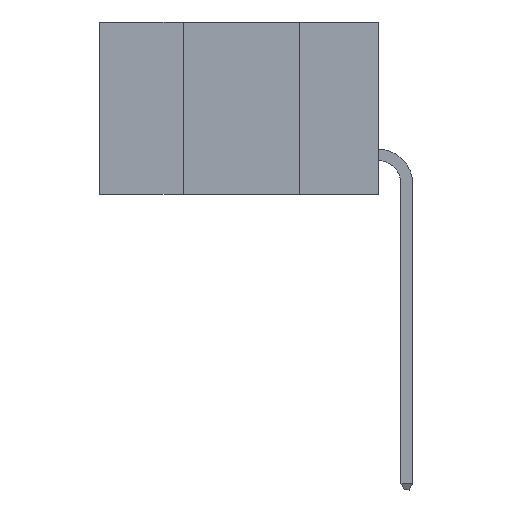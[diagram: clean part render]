
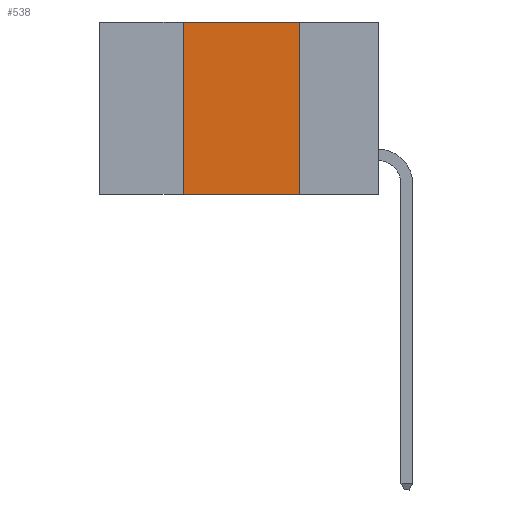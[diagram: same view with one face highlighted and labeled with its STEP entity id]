
A CAD part, left-side view. The second image highlights one B-rep face of the part: STEP entity #538.
In plain terms, the highlighted planar face has unit normal (-1, 0, 0).
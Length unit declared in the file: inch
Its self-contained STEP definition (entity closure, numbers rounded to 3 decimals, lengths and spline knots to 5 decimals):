
#421 = EDGE_LOOP ( 'NONE', ( #5904, #5609, #13743, #13166 ) ) ;
#538 = ADVANCED_FACE ( 'NONE', ( #7752 ), #2664, .F. ) ;
#1612 = CARTESIAN_POINT ( 'NONE',  ( 0., 0.17, 0. ) ) ;
#2026 = VECTOR ( 'NONE', #13033, 39.37008 ) ;
#2372 = DIRECTION ( 'NONE',  ( 0., -1., 0. ) ) ;
#2664 = PLANE ( 'NONE',  #4164 ) ;
#3254 = VERTEX_POINT ( 'NONE', #11123 ) ;
#3627 = EDGE_CURVE ( 'NONE', #9568, #3254, #14555, .T. ) ;
#3674 = DIRECTION ( 'NONE',  ( 0., 0., -1. ) ) ;
#4120 = VECTOR ( 'NONE', #5098, 39.37008 ) ;
#4164 = AXIS2_PLACEMENT_3D ( 'NONE', #4630, #5545, #3674 ) ;
#4630 = CARTESIAN_POINT ( 'NONE',  ( 0., 0.6, 0. ) ) ;
#5098 = DIRECTION ( 'NONE',  ( 0., 0., -1. ) ) ;
#5545 = DIRECTION ( 'NONE',  ( 1., 0., 0. ) ) ;
#5562 = DIRECTION ( 'NONE',  ( 0., -1., 0. ) ) ;
#5609 = ORIENTED_EDGE ( 'NONE', *, *, #7750, .F. ) ;
#5904 = ORIENTED_EDGE ( 'NONE', *, *, #6982, .F. ) ;
#6234 = EDGE_CURVE ( 'NONE', #9568, #12731, #7183, .T. ) ;
#6982 = EDGE_CURVE ( 'NONE', #8669, #12731, #11295, .T. ) ;
#7183 = LINE ( 'NONE', #10643, #13020 ) ;
#7711 = CARTESIAN_POINT ( 'NONE',  ( 0., 0.42, -0.37 ) ) ;
#7750 = EDGE_CURVE ( 'NONE', #3254, #8669, #12399, .T. ) ;
#7752 = FACE_OUTER_BOUND ( 'NONE', #421, .T. ) ;
#7770 = CARTESIAN_POINT ( 'NONE',  ( 0., 0.42, 0. ) ) ;
#8669 = VERTEX_POINT ( 'NONE', #11096 ) ;
#9568 = VERTEX_POINT ( 'NONE', #7711 ) ;
#10643 = CARTESIAN_POINT ( 'NONE',  ( 0., 0.6, -0.37 ) ) ;
#10665 = CARTESIAN_POINT ( 'NONE',  ( 0., 0.17, -0.37 ) ) ;
#10879 = CARTESIAN_POINT ( 'NONE',  ( 0., 0.6, 0. ) ) ;
#11096 = CARTESIAN_POINT ( 'NONE',  ( 0., 0.17, 0. ) ) ;
#11123 = CARTESIAN_POINT ( 'NONE',  ( 0., 0.42, 0. ) ) ;
#11295 = LINE ( 'NONE', #1612, #4120 ) ;
#12399 = LINE ( 'NONE', #10879, #15186 ) ;
#12731 = VERTEX_POINT ( 'NONE', #10665 ) ;
#13020 = VECTOR ( 'NONE', #5562, 39.37008 ) ;
#13033 = DIRECTION ( 'NONE',  ( 0., 0., 1. ) ) ;
#13166 = ORIENTED_EDGE ( 'NONE', *, *, #6234, .T. ) ;
#13743 = ORIENTED_EDGE ( 'NONE', *, *, #3627, .F. ) ;
#14555 = LINE ( 'NONE', #7770, #2026 ) ;
#15186 = VECTOR ( 'NONE', #2372, 39.37008 ) ;
